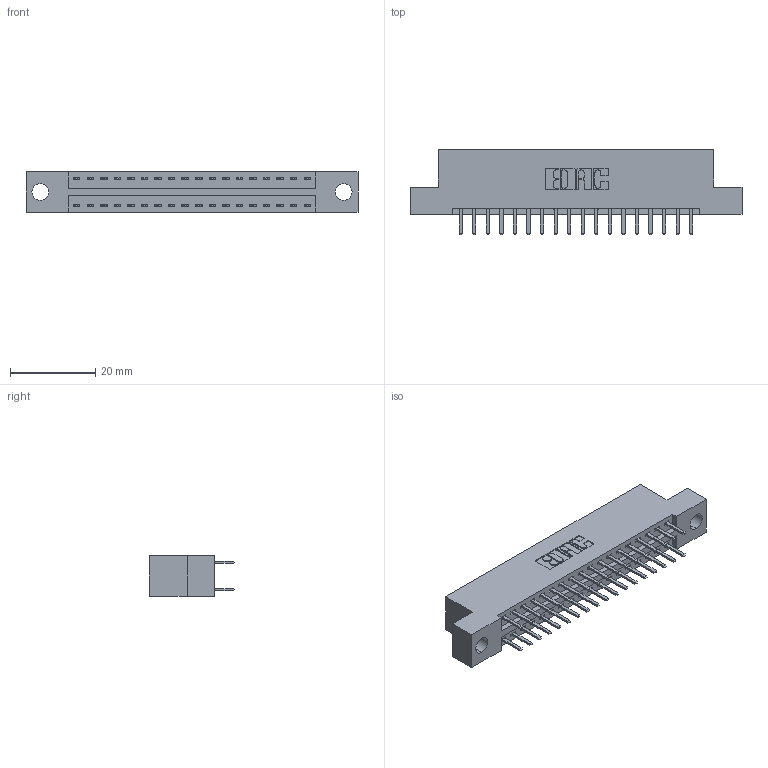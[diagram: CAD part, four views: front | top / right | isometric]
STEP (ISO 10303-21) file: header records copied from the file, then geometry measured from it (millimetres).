
FILE_DESCRIPTION (( 'STEP AP203' ), '1' );
FILE_NAME ('346-036-520-204.STEP', '2022-05-19T20:57:05', ( '' ), ( '' ), 'SwSTEP 2.0', 'SolidWorks 2020', '' );
FILE_SCHEMA (( 'CONFIG_CONTROL_DESIGN' ));
Length unit declared in the file: inch
Products named in the file (3): 345-292-001_345-293-120; 346-036-520-204; 346 Part_Flush Mounting Lugs - 0.156 Dia-TH
Assembly tree (37 placements, depth 2):
  346-036-520-204
    346 Part_Flush Mounting Lugs - 0.156 Dia-TH
    345-292-001_345-293-120  x36
Bounding box: 77.72 x 20.02 x 9.4 mm (x, y, z)
Volume: 7270.9 mm3; surface area: 9427.9 mm2
Topology: 37 solids, 37 shells, 2152 faces, 6233 edges, 4058 vertices
Faces by surface type: plane 1422, cylinder 730
Entity records: 15511 total; most frequent: CARTESIAN_POINT 2606, ORIENTED_EDGE 2526, DIRECTION 2335, EDGE_CURVE 1263, LINE 1055, VECTOR 1055, VERTEX_POINT 838, AXIS2_PLACEMENT_3D 640
